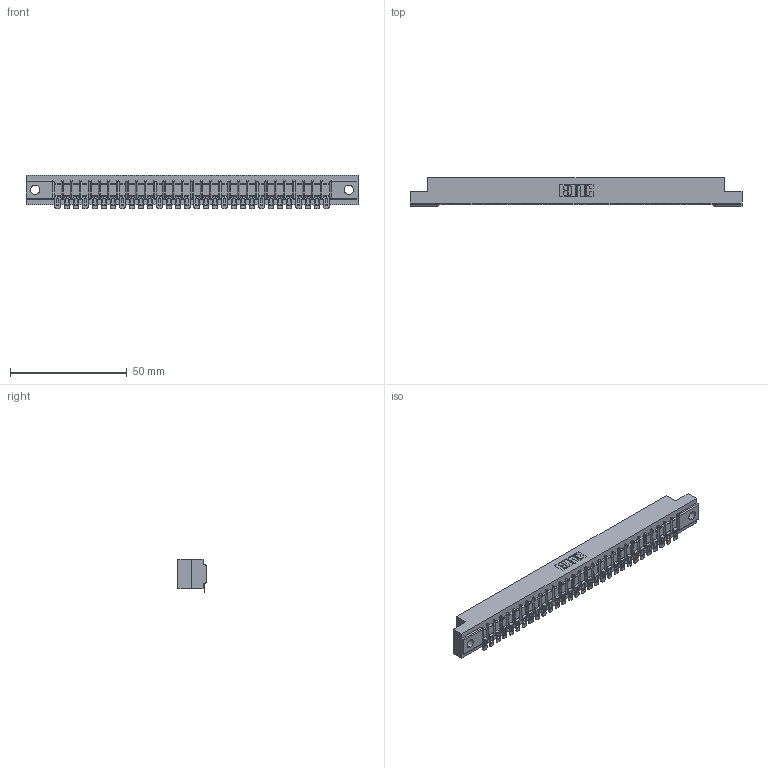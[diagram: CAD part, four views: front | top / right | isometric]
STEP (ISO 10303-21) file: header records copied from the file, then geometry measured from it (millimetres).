
FILE_DESCRIPTION (( 'STEP AP203' ), '1' );
FILE_NAME ('307-030-454-104.STEP', '2020-09-28T12:12:18', ( '' ), ( '' ), 'SwSTEP 2.0', 'SolidWorks 2020', '' );
FILE_SCHEMA (( 'CONFIG_CONTROL_DESIGN' ));
Length unit declared in the file: inch
Products named in the file (3): 307 Part_.156 Dia Mounting Holes; 307-030-454-104; 307-290-002_554
Assembly tree (31 placements, depth 2):
  307-030-454-104
    307 Part_.156 Dia Mounting Holes
    307-290-002_554  x30
Bounding box: 141.88 x 12.01 x 14.52 mm (x, y, z)
Volume: 14998.8 mm3; surface area: 18547.6 mm2
Topology: 31 solids, 31 shells, 2593 faces, 7949 edges, 5214 vertices
Faces by surface type: plane 1464, cylinder 1067, sphere 62
Entity records: 28581 total; most frequent: CARTESIAN_POINT 4824, ORIENTED_EDGE 4812, DIRECTION 4690, EDGE_CURVE 2406, VECTOR 1838, LINE 1838, VERTEX_POINT 1560, AXIS2_PLACEMENT_3D 1426
